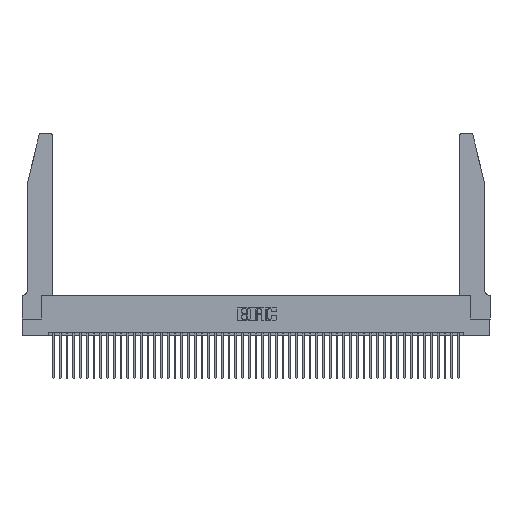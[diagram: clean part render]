
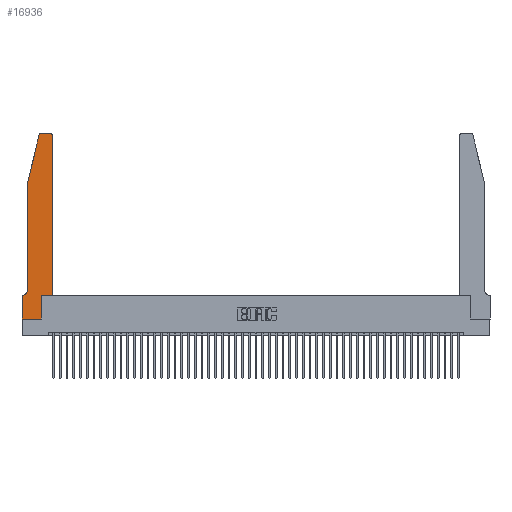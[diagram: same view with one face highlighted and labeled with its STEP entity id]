
A CAD part, top view. The second image highlights one B-rep face of the part: STEP entity #16936.
In plain terms, the highlighted planar face has unit normal (0, 0, 1).
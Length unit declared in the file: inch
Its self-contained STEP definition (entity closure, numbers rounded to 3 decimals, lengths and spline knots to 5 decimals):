
#63 = VERTEX_POINT ( 'NONE', #3407 ) ;
#569 = CIRCLE ( 'NONE', #5072, 0.03 ) ;
#1303 = VERTEX_POINT ( 'NONE', #17422 ) ;
#2404 = CARTESIAN_POINT ( 'NONE',  ( 0.4505, 0.35, 0.37 ) ) ;
#2676 = VECTOR ( 'NONE', #43931, 39.37008 ) ;
#3407 = CARTESIAN_POINT ( 'NONE',  ( 0.0755, 2., 0.37 ) ) ;
#3564 = CARTESIAN_POINT ( 'NONE',  ( 0.4205, 2.72, 0.37 ) ) ;
#3939 = LINE ( 'NONE', #21063, #2676 ) ;
#3972 = AXIS2_PLACEMENT_3D ( 'NONE', #10330, #37264, #14291 ) ;
#4279 = LINE ( 'NONE', #25621, #34112 ) ;
#5072 = AXIS2_PLACEMENT_3D ( 'NONE', #28799, #5460, #32659 ) ;
#5210 = EDGE_CURVE ( 'NONE', #26230, #11790, #12177, .T. ) ;
#5460 = DIRECTION ( 'NONE',  ( 0., 0., 1. ) ) ;
#6099 = LINE ( 'NONE', #12806, #25681 ) ;
#6438 = VECTOR ( 'NONE', #23248, 39.37008 ) ;
#7431 = EDGE_CURVE ( 'NONE', #13030, #27064, #33740, .T. ) ;
#7580 = ORIENTED_EDGE ( 'NONE', *, *, #46713, .T. ) ;
#7583 = DIRECTION ( 'NONE',  ( 1., 0., 0. ) ) ;
#8791 = CARTESIAN_POINT ( 'NONE',  ( 0.4205, 2.75, 0.37 ) ) ;
#8945 = LINE ( 'NONE', #49590, #18147 ) ;
#10330 = CARTESIAN_POINT ( 'NONE',  ( 0.0055, 0.42, 0.37 ) ) ;
#11790 = VERTEX_POINT ( 'NONE', #19477 ) ;
#12159 = CARTESIAN_POINT ( 'NONE',  ( 0.2865, 0., 0.37 ) ) ;
#12177 = LINE ( 'NONE', #2404, #31503 ) ;
#12806 = CARTESIAN_POINT ( 'NONE',  ( 0., 0., 0.37 ) ) ;
#13012 = ORIENTED_EDGE ( 'NONE', *, *, #32468, .T. ) ;
#13030 = VERTEX_POINT ( 'NONE', #38452 ) ;
#13114 = DIRECTION ( 'NONE',  ( -1., 0., 0. ) ) ;
#13170 = CARTESIAN_POINT ( 'NONE',  ( 0.2865, 0.35, 0.37 ) ) ;
#13270 = EDGE_CURVE ( 'NONE', #33387, #14611, #3939, .T. ) ;
#13871 = DIRECTION ( 'NONE',  ( 0., 0., 1. ) ) ;
#14246 = AXIS2_PLACEMENT_3D ( 'NONE', #3564, #30818, #7583 ) ;
#14291 = DIRECTION ( 'NONE',  ( -1., 0., 0. ) ) ;
#14611 = VERTEX_POINT ( 'NONE', #13170 ) ;
#15369 = EDGE_CURVE ( 'NONE', #28311, #40608, #569, .T. ) ;
#15628 = VECTOR ( 'NONE', #43799, 39.37008 ) ;
#15830 = CARTESIAN_POINT ( 'NONE',  ( 0.284, 2.75, 0.37 ) ) ;
#16730 = DIRECTION ( 'NONE',  ( 1., 0., 0. ) ) ;
#16928 = LINE ( 'NONE', #38462, #6438 ) ;
#16936 = ADVANCED_FACE ( 'NONE', ( #41376 ), #36872, .T. ) ;
#17422 = CARTESIAN_POINT ( 'NONE',  ( 0.0755, 0.42, 0.37 ) ) ;
#18147 = VECTOR ( 'NONE', #30657, 39.37008 ) ;
#18245 = ORIENTED_EDGE ( 'NONE', *, *, #49899, .T. ) ;
#19255 = CARTESIAN_POINT ( 'NONE',  ( 0., 0., 0.37 ) ) ;
#19477 = CARTESIAN_POINT ( 'NONE',  ( 0.4505, 2.72, 0.37 ) ) ;
#20956 = VERTEX_POINT ( 'NONE', #8791 ) ;
#21063 = CARTESIAN_POINT ( 'NONE',  ( 0.2865, 0.35, 0.37 ) ) ;
#21984 = CARTESIAN_POINT ( 'NONE',  ( 0.0755, 2., 0.37 ) ) ;
#23167 = ORIENTED_EDGE ( 'NONE', *, *, #7431, .T. ) ;
#23248 = DIRECTION ( 'NONE',  ( 0., -1., 0. ) ) ;
#23251 = CARTESIAN_POINT ( 'NONE',  ( 0.4505, 0.35, 0.37 ) ) ;
#23505 = VECTOR ( 'NONE', #13114, 39.37008 ) ;
#24777 = AXIS2_PLACEMENT_3D ( 'NONE', #40495, #13871, #40661 ) ;
#25621 = CARTESIAN_POINT ( 'NONE',  ( 0.4505, 0.35, 0.37 ) ) ;
#25681 = VECTOR ( 'NONE', #16730, 39.37008 ) ;
#25700 = VERTEX_POINT ( 'NONE', #19255 ) ;
#26230 = VERTEX_POINT ( 'NONE', #23251 ) ;
#26671 = EDGE_CURVE ( 'NONE', #1303, #13030, #31095, .T. ) ;
#27064 = VERTEX_POINT ( 'NONE', #28073 ) ;
#27138 = VECTOR ( 'NONE', #41009, 39.37008 ) ;
#27334 = EDGE_LOOP ( 'NONE', ( #34099, #29892, #46087, #34851, #37108, #23167, #18245, #7580, #28124, #13012, #47167, #33575 ) ) ;
#28073 = CARTESIAN_POINT ( 'NONE',  ( 0., 0.35, 0.37 ) ) ;
#28124 = ORIENTED_EDGE ( 'NONE', *, *, #13270, .T. ) ;
#28311 = VERTEX_POINT ( 'NONE', #15830 ) ;
#28338 = LINE ( 'NONE', #21984, #27138 ) ;
#28799 = CARTESIAN_POINT ( 'NONE',  ( 0.284, 2.72, 0.37 ) ) ;
#29892 = ORIENTED_EDGE ( 'NONE', *, *, #15369, .T. ) ;
#30657 = DIRECTION ( 'NONE',  ( -1., 0., 0. ) ) ;
#30818 = DIRECTION ( 'NONE',  ( 0., 0., 1. ) ) ;
#31095 = CIRCLE ( 'NONE', #3972, 0.07 ) ;
#31503 = VECTOR ( 'NONE', #41006, 39.37008 ) ;
#32468 = EDGE_CURVE ( 'NONE', #14611, #26230, #4279, .T. ) ;
#32659 = DIRECTION ( 'NONE',  ( 1., 0., 0. ) ) ;
#33387 = VERTEX_POINT ( 'NONE', #12159 ) ;
#33575 = ORIENTED_EDGE ( 'NONE', *, *, #48965, .T. ) ;
#33740 = LINE ( 'NONE', #36163, #23505 ) ;
#34099 = ORIENTED_EDGE ( 'NONE', *, *, #48912, .T. ) ;
#34112 = VECTOR ( 'NONE', #48427, 39.37008 ) ;
#34851 = ORIENTED_EDGE ( 'NONE', *, *, #48973, .T. ) ;
#36074 = LINE ( 'NONE', #47619, #15628 ) ;
#36163 = CARTESIAN_POINT ( 'NONE',  ( 0.0755, 0.35, 0.37 ) ) ;
#36872 = PLANE ( 'NONE',  #24777 ) ;
#37108 = ORIENTED_EDGE ( 'NONE', *, *, #26671, .T. ) ;
#37264 = DIRECTION ( 'NONE',  ( 0., 0., -1. ) ) ;
#37308 = CIRCLE ( 'NONE', #14246, 0.03 ) ;
#38452 = CARTESIAN_POINT ( 'NONE',  ( 0.0055, 0.35, 0.37 ) ) ;
#38462 = CARTESIAN_POINT ( 'NONE',  ( 0.0755, 2., 0.37 ) ) ;
#40495 = CARTESIAN_POINT ( 'NONE',  ( 0., 0.35, 0.37 ) ) ;
#40608 = VERTEX_POINT ( 'NONE', #44209 ) ;
#40661 = DIRECTION ( 'NONE',  ( 1., 0., 0. ) ) ;
#41006 = DIRECTION ( 'NONE',  ( 0., 1., 0. ) ) ;
#41009 = DIRECTION ( 'NONE',  ( -0.239, -0.971, 0. ) ) ;
#41376 = FACE_OUTER_BOUND ( 'NONE', #27334, .T. ) ;
#43799 = DIRECTION ( 'NONE',  ( 0., -1., 0. ) ) ;
#43931 = DIRECTION ( 'NONE',  ( 0., 1., 0. ) ) ;
#44209 = CARTESIAN_POINT ( 'NONE',  ( 0.25487, 2.72718, 0.37 ) ) ;
#46087 = ORIENTED_EDGE ( 'NONE', *, *, #49407, .T. ) ;
#46713 = EDGE_CURVE ( 'NONE', #25700, #33387, #6099, .T. ) ;
#47167 = ORIENTED_EDGE ( 'NONE', *, *, #5210, .T. ) ;
#47619 = CARTESIAN_POINT ( 'NONE',  ( 0., 0., 0.37 ) ) ;
#48427 = DIRECTION ( 'NONE',  ( 1., 0., 0. ) ) ;
#48912 = EDGE_CURVE ( 'NONE', #20956, #28311, #8945, .T. ) ;
#48965 = EDGE_CURVE ( 'NONE', #11790, #20956, #37308, .T. ) ;
#48973 = EDGE_CURVE ( 'NONE', #63, #1303, #16928, .T. ) ;
#49407 = EDGE_CURVE ( 'NONE', #40608, #63, #28338, .T. ) ;
#49590 = CARTESIAN_POINT ( 'NONE',  ( 0.2605, 2.75, 0.37 ) ) ;
#49899 = EDGE_CURVE ( 'NONE', #27064, #25700, #36074, .T. ) ;
